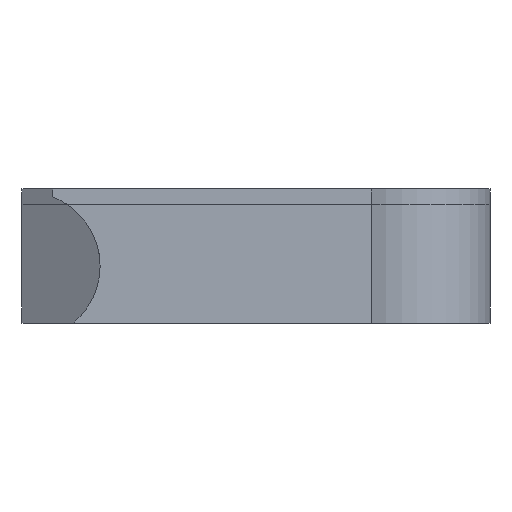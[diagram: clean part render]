
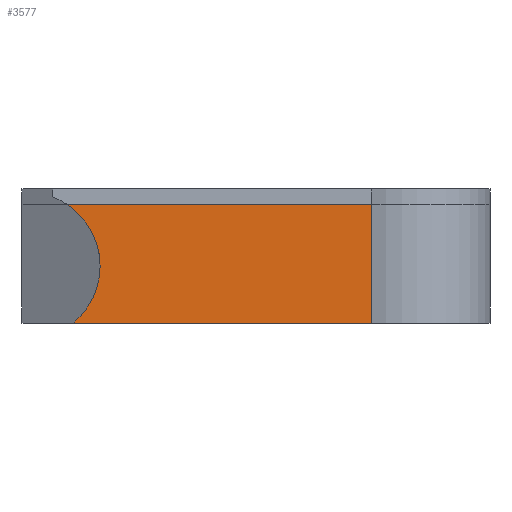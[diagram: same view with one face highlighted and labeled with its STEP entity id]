
A CAD part, left-side view. The second image highlights one B-rep face of the part: STEP entity #3577.
In plain terms, the highlighted planar face has unit normal (-1, 0, 0).
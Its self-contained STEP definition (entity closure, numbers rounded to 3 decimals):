
#543 = CYLINDRICAL_SURFACE('',#544,5.);
#544 = AXIS2_PLACEMENT_3D('',#545,#546,#547);
#545 = CARTESIAN_POINT('',(-13.,23.3,3.85));
#546 = DIRECTION('',(-1.,0.,0.));
#547 = DIRECTION('',(0.,-1.,0.));
#620 = PLANE('',#621);
#621 = AXIS2_PLACEMENT_3D('',#622,#623,#624);
#622 = CARTESIAN_POINT('',(0.,0.,0.));
#623 = DIRECTION('',(0.,0.,1.));
#624 = DIRECTION('',(1.,0.,0.));
#1806 = VERTEX_POINT('',#1807);
#1807 = CARTESIAN_POINT('',(-13.,18.3,3.85));
#1823 = CYLINDRICAL_SURFACE('',#1824,5.);
#1824 = AXIS2_PLACEMENT_3D('',#1825,#1826,#1827);
#1825 = CARTESIAN_POINT('',(-13.,23.3,3.85));
#1826 = DIRECTION('',(-1.,0.,0.));
#1827 = DIRECTION('',(0.,-1.,0.));
#1835 = EDGE_CURVE('',#1836,#1806,#1838,.T.);
#1836 = VERTEX_POINT('',#1837);
#1837 = CARTESIAN_POINT('',(-13.,20.11,0.));
#1838 = SURFACE_CURVE('',#1839,(#1844,#1851),.PCURVE_S1.);
#1839 = CIRCLE('',#1840,5.);
#1840 = AXIS2_PLACEMENT_3D('',#1841,#1842,#1843);
#1841 = CARTESIAN_POINT('',(-13.,23.3,3.85));
#1842 = DIRECTION('',(-1.,0.,0.));
#1843 = DIRECTION('',(0.,-1.,0.));
#1844 = PCURVE('',#543,#1845);
#1845 = DEFINITIONAL_REPRESENTATION('',(#1846),#1850);
#1846 = LINE('',#1847,#1848);
#1847 = CARTESIAN_POINT('',(0.,0.));
#1848 = VECTOR('',#1849,1.);
#1849 = DIRECTION('',(1.,0.));
#1850 = ( GEOMETRIC_REPRESENTATION_CONTEXT(2) 
PARAMETRIC_REPRESENTATION_CONTEXT() REPRESENTATION_CONTEXT('2D SPACE',''
  ) );
#1851 = PCURVE('',#1852,#1857);
#1852 = PLANE('',#1853);
#1853 = AXIS2_PLACEMENT_3D('',#1854,#1855,#1856);
#1854 = CARTESIAN_POINT('',(-13.,0.,0.));
#1855 = DIRECTION('',(-1.,0.,0.));
#1856 = DIRECTION('',(0.,1.,0.));
#1857 = DEFINITIONAL_REPRESENTATION('',(#1858),#1862);
#1858 = CIRCLE('',#1859,5.);
#1859 = AXIS2_PLACEMENT_2D('',#1860,#1861);
#1860 = CARTESIAN_POINT('',(23.3,-3.85));
#1861 = DIRECTION('',(-1.,0.));
#1862 = ( GEOMETRIC_REPRESENTATION_CONTEXT(2) 
PARAMETRIC_REPRESENTATION_CONTEXT() REPRESENTATION_CONTEXT('2D SPACE',''
  ) );
#2046 = PLANE('',#2047);
#2047 = AXIS2_PLACEMENT_3D('',#2048,#2049,#2050);
#2048 = CARTESIAN_POINT('',(0.,0.,0.));
#2049 = DIRECTION('',(0.,-1.,0.));
#2050 = DIRECTION('',(-1.,0.,0.));
#2064 = EDGE_CURVE('',#2065,#1836,#2067,.T.);
#2065 = VERTEX_POINT('',#2066);
#2066 = CARTESIAN_POINT('',(-13.,0.,0.));
#2067 = SURFACE_CURVE('',#2068,(#2072,#2079),.PCURVE_S1.);
#2068 = LINE('',#2069,#2070);
#2069 = CARTESIAN_POINT('',(-13.,0.,0.));
#2070 = VECTOR('',#2071,1.);
#2071 = DIRECTION('',(0.,1.,0.));
#2072 = PCURVE('',#620,#2073);
#2073 = DEFINITIONAL_REPRESENTATION('',(#2074),#2078);
#2074 = LINE('',#2075,#2076);
#2075 = CARTESIAN_POINT('',(-13.,0.));
#2076 = VECTOR('',#2077,1.);
#2077 = DIRECTION('',(0.,1.));
#2078 = ( GEOMETRIC_REPRESENTATION_CONTEXT(2) 
PARAMETRIC_REPRESENTATION_CONTEXT() REPRESENTATION_CONTEXT('2D SPACE',''
  ) );
#2079 = PCURVE('',#1852,#2080);
#2080 = DEFINITIONAL_REPRESENTATION('',(#2081),#2085);
#2081 = LINE('',#2082,#2083);
#2082 = CARTESIAN_POINT('',(0.,0.));
#2083 = VECTOR('',#2084,1.);
#2084 = DIRECTION('',(1.,0.));
#2085 = ( GEOMETRIC_REPRESENTATION_CONTEXT(2) 
PARAMETRIC_REPRESENTATION_CONTEXT() REPRESENTATION_CONTEXT('2D SPACE',''
  ) );
#2112 = VERTEX_POINT('',#2113);
#2113 = CARTESIAN_POINT('',(-13.,0.,8.));
#2150 = PLANE('',#2151);
#2151 = AXIS2_PLACEMENT_3D('',#2152,#2153,#2154);
#2152 = CARTESIAN_POINT('',(-13.,23.564,8.));
#2153 = DIRECTION('',(1.,0.,0.));
#2154 = DIRECTION('',(0.,-1.,0.));
#3449 = EDGE_CURVE('',#1806,#3450,#3452,.T.);
#3450 = VERTEX_POINT('',#3451);
#3451 = CARTESIAN_POINT('',(-13.,20.511,8.));
#3452 = SURFACE_CURVE('',#3453,(#3458,#3465),.PCURVE_S1.);
#3453 = CIRCLE('',#3454,5.);
#3454 = AXIS2_PLACEMENT_3D('',#3455,#3456,#3457);
#3455 = CARTESIAN_POINT('',(-13.,23.3,3.85));
#3456 = DIRECTION('',(-1.,0.,0.));
#3457 = DIRECTION('',(0.,-1.,0.));
#3458 = PCURVE('',#1823,#3459);
#3459 = DEFINITIONAL_REPRESENTATION('',(#3460),#3464);
#3460 = LINE('',#3461,#3462);
#3461 = CARTESIAN_POINT('',(0.,0.));
#3462 = VECTOR('',#3463,1.);
#3463 = DIRECTION('',(1.,0.));
#3464 = ( GEOMETRIC_REPRESENTATION_CONTEXT(2) 
PARAMETRIC_REPRESENTATION_CONTEXT() REPRESENTATION_CONTEXT('2D SPACE',''
  ) );
#3465 = PCURVE('',#1852,#3466);
#3466 = DEFINITIONAL_REPRESENTATION('',(#3467),#3471);
#3467 = CIRCLE('',#3468,5.);
#3468 = AXIS2_PLACEMENT_2D('',#3469,#3470);
#3469 = CARTESIAN_POINT('',(23.3,-3.85));
#3470 = DIRECTION('',(-1.,0.));
#3471 = ( GEOMETRIC_REPRESENTATION_CONTEXT(2) 
PARAMETRIC_REPRESENTATION_CONTEXT() REPRESENTATION_CONTEXT('2D SPACE',''
  ) );
#3577 = ADVANCED_FACE('',(#3578),#1852,.T.);
#3578 = FACE_BOUND('',#3579,.T.);
#3579 = EDGE_LOOP('',(#3580,#3581,#3582,#3603,#3624));
#3580 = ORIENTED_EDGE('',*,*,#1835,.F.);
#3581 = ORIENTED_EDGE('',*,*,#2064,.F.);
#3582 = ORIENTED_EDGE('',*,*,#3583,.T.);
#3583 = EDGE_CURVE('',#2065,#2112,#3584,.T.);
#3584 = SURFACE_CURVE('',#3585,(#3589,#3596),.PCURVE_S1.);
#3585 = LINE('',#3586,#3587);
#3586 = CARTESIAN_POINT('',(-13.,0.,0.));
#3587 = VECTOR('',#3588,1.);
#3588 = DIRECTION('',(0.,0.,1.));
#3589 = PCURVE('',#1852,#3590);
#3590 = DEFINITIONAL_REPRESENTATION('',(#3591),#3595);
#3591 = LINE('',#3592,#3593);
#3592 = CARTESIAN_POINT('',(0.,0.));
#3593 = VECTOR('',#3594,1.);
#3594 = DIRECTION('',(0.,-1.));
#3595 = ( GEOMETRIC_REPRESENTATION_CONTEXT(2) 
PARAMETRIC_REPRESENTATION_CONTEXT() REPRESENTATION_CONTEXT('2D SPACE',''
  ) );
#3596 = PCURVE('',#2046,#3597);
#3597 = DEFINITIONAL_REPRESENTATION('',(#3598),#3602);
#3598 = LINE('',#3599,#3600);
#3599 = CARTESIAN_POINT('',(13.,0.));
#3600 = VECTOR('',#3601,1.);
#3601 = DIRECTION('',(0.,-1.));
#3602 = ( GEOMETRIC_REPRESENTATION_CONTEXT(2) 
PARAMETRIC_REPRESENTATION_CONTEXT() REPRESENTATION_CONTEXT('2D SPACE',''
  ) );
#3603 = ORIENTED_EDGE('',*,*,#3604,.F.);
#3604 = EDGE_CURVE('',#3450,#2112,#3605,.T.);
#3605 = SURFACE_CURVE('',#3606,(#3610,#3617),.PCURVE_S1.);
#3606 = LINE('',#3607,#3608);
#3607 = CARTESIAN_POINT('',(-13.,23.564,8.));
#3608 = VECTOR('',#3609,1.);
#3609 = DIRECTION('',(0.,-1.,0.));
#3610 = PCURVE('',#1852,#3611);
#3611 = DEFINITIONAL_REPRESENTATION('',(#3612),#3616);
#3612 = LINE('',#3613,#3614);
#3613 = CARTESIAN_POINT('',(23.564,-8.));
#3614 = VECTOR('',#3615,1.);
#3615 = DIRECTION('',(-1.,0.));
#3616 = ( GEOMETRIC_REPRESENTATION_CONTEXT(2) 
PARAMETRIC_REPRESENTATION_CONTEXT() REPRESENTATION_CONTEXT('2D SPACE',''
  ) );
#3617 = PCURVE('',#2150,#3618);
#3618 = DEFINITIONAL_REPRESENTATION('',(#3619),#3623);
#3619 = LINE('',#3620,#3621);
#3620 = CARTESIAN_POINT('',(0.,0.));
#3621 = VECTOR('',#3622,1.);
#3622 = DIRECTION('',(1.,0.));
#3623 = ( GEOMETRIC_REPRESENTATION_CONTEXT(2) 
PARAMETRIC_REPRESENTATION_CONTEXT() REPRESENTATION_CONTEXT('2D SPACE',''
  ) );
#3624 = ORIENTED_EDGE('',*,*,#3449,.F.);
